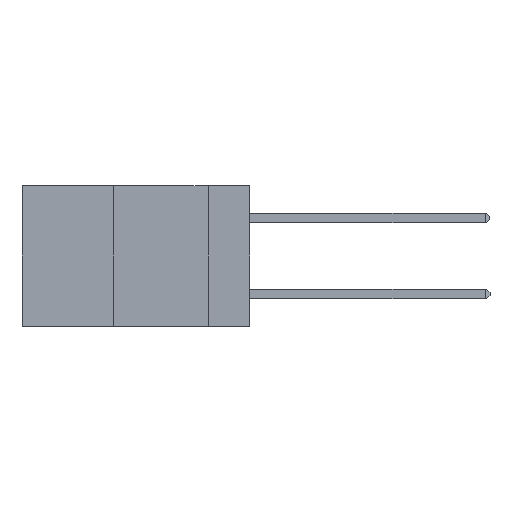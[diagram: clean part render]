
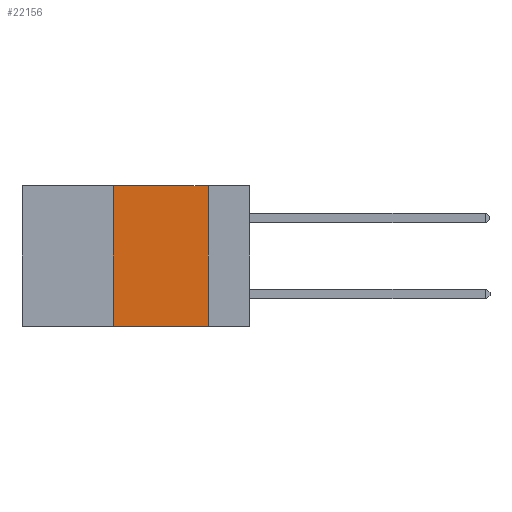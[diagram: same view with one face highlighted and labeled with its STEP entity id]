
A CAD part, left-side view. The second image highlights one B-rep face of the part: STEP entity #22156.
In plain terms, the highlighted planar face has unit normal (-1, 0, 0).
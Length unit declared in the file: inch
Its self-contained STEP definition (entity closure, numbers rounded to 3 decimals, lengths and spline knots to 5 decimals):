
#466 = VECTOR ( 'NONE', #7722, 39.37008 ) ;
#700 = AXIS2_PLACEMENT_3D ( 'NONE', #2950, #12677, #16246 ) ;
#786 = LINE ( 'NONE', #16569, #20824 ) ;
#1406 = DIRECTION ( 'NONE',  ( 0., -1., 0. ) ) ;
#1470 = VECTOR ( 'NONE', #11427, 39.37008 ) ;
#1497 = CARTESIAN_POINT ( 'NONE',  ( 0., 0.11, -0.37 ) ) ;
#2950 = CARTESIAN_POINT ( 'NONE',  ( 0., 0.6, 0. ) ) ;
#3438 = VERTEX_POINT ( 'NONE', #18278 ) ;
#3781 = VERTEX_POINT ( 'NONE', #9213 ) ;
#5923 = VERTEX_POINT ( 'NONE', #23682 ) ;
#6354 = CARTESIAN_POINT ( 'NONE',  ( 0., 0.6, -0.37 ) ) ;
#7166 = ORIENTED_EDGE ( 'NONE', *, *, #24582, .T. ) ;
#7722 = DIRECTION ( 'NONE',  ( 0., -1., 0. ) ) ;
#8927 = EDGE_LOOP ( 'NONE', ( #22032, #24958, #19226, #7166 ) ) ;
#9213 = CARTESIAN_POINT ( 'NONE',  ( 0., 0.36, -0.37 ) ) ;
#9597 = EDGE_CURVE ( 'NONE', #3438, #16820, #786, .T. ) ;
#10893 = LINE ( 'NONE', #16922, #13315 ) ;
#11427 = DIRECTION ( 'NONE',  ( 0., 0., 1. ) ) ;
#11566 = FACE_OUTER_BOUND ( 'NONE', #8927, .T. ) ;
#12677 = DIRECTION ( 'NONE',  ( 1., 0., 0. ) ) ;
#13315 = VECTOR ( 'NONE', #1406, 39.37008 ) ;
#14729 = LINE ( 'NONE', #6354, #466 ) ;
#15989 = PLANE ( 'NONE',  #700 ) ;
#16246 = DIRECTION ( 'NONE',  ( 0., 0., -1. ) ) ;
#16569 = CARTESIAN_POINT ( 'NONE',  ( 0., 0.11, 0. ) ) ;
#16820 = VERTEX_POINT ( 'NONE', #1497 ) ;
#16922 = CARTESIAN_POINT ( 'NONE',  ( 0., 0.6, 0. ) ) ;
#17090 = EDGE_CURVE ( 'NONE', #5923, #3438, #10893, .T. ) ;
#18147 = EDGE_CURVE ( 'NONE', #3781, #5923, #21203, .T. ) ;
#18278 = CARTESIAN_POINT ( 'NONE',  ( 0., 0.11, 0. ) ) ;
#19021 = DIRECTION ( 'NONE',  ( 0., 0., -1. ) ) ;
#19226 = ORIENTED_EDGE ( 'NONE', *, *, #18147, .F. ) ;
#19344 = CARTESIAN_POINT ( 'NONE',  ( 0., 0.36, 0. ) ) ;
#20824 = VECTOR ( 'NONE', #19021, 39.37008 ) ;
#21203 = LINE ( 'NONE', #19344, #1470 ) ;
#22032 = ORIENTED_EDGE ( 'NONE', *, *, #9597, .F. ) ;
#22156 = ADVANCED_FACE ( 'NONE', ( #11566 ), #15989, .F. ) ;
#23682 = CARTESIAN_POINT ( 'NONE',  ( 0., 0.36, 0. ) ) ;
#24582 = EDGE_CURVE ( 'NONE', #3781, #16820, #14729, .T. ) ;
#24958 = ORIENTED_EDGE ( 'NONE', *, *, #17090, .F. ) ;
